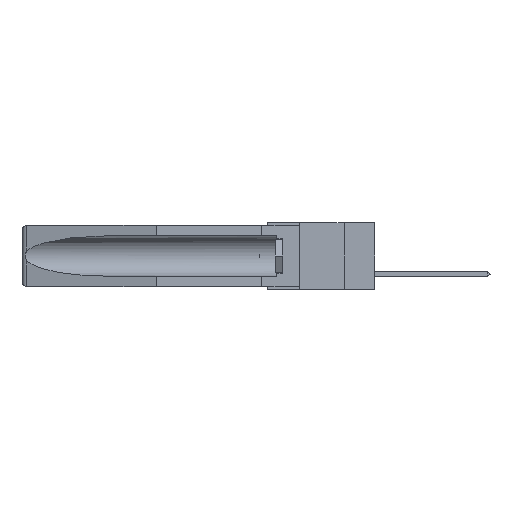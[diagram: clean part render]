
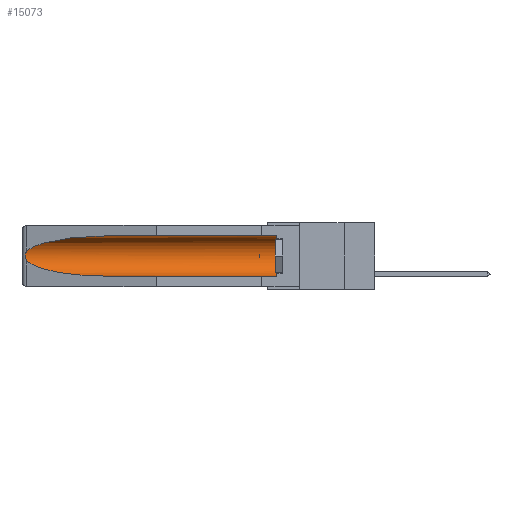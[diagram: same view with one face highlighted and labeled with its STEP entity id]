
A CAD part, left-side view. The second image highlights one B-rep face of the part: STEP entity #15073.
In plain terms, the highlighted cylindrical face has radius 2.857 mm (diameter 5.715 mm), a partial arc.
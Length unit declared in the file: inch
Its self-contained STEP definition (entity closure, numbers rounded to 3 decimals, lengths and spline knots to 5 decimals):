
#149 = CARTESIAN_POINT ( 'NONE',  ( 0.25451, 1.48313, -0.24835 ) ) ;
#455 =( BOUNDED_CURVE ( )  B_SPLINE_CURVE ( 3, ( #33222, #30406, #4039, #22581 ),
 .UNSPECIFIED., .F., .F. ) 
 B_SPLINE_CURVE_WITH_KNOTS ( ( 4, 4 ),
 ( 4.71239, 6.08839 ),
 .UNSPECIFIED. ) 
 CURVE ( )  GEOMETRIC_REPRESENTATION_ITEM ( )  RATIONAL_B_SPLINE_CURVE ( ( 1., 0.848, 0.848, 1. ) ) 
 REPRESENTATION_ITEM ( '' )  );
#1228 = VECTOR ( 'NONE', #14519, 39.37008 ) ;
#1264 = LINE ( 'NONE', #25071, #1228 ) ;
#1366 = VERTEX_POINT ( 'NONE', #9580 ) ;
#1569 = CARTESIAN_POINT ( 'NONE',  ( 0.26597, 1.5296, -0.19026 ) ) ;
#2656 = CARTESIAN_POINT ( 'NONE',  ( 0.155, 1.07973, -0.284 ) ) ;
#2924 = VERTEX_POINT ( 'NONE', #24906 ) ;
#3995 = CARTESIAN_POINT ( 'NONE',  ( 0.26655, 1.53094, -0.18657 ) ) ;
#4039 = CARTESIAN_POINT ( 'NONE',  ( 0.25451, 1.48313, -0.09465 ) ) ;
#4229 = CARTESIAN_POINT ( 'NONE',  ( 0.26537, 1.52718, -0.19328 ) ) ;
#4507 = ORIENTED_EDGE ( 'NONE', *, *, #25026, .T. ) ;
#4706 = EDGE_CURVE ( 'NONE', #17522, #2924, #455, .T. ) ;
#6212 = CARTESIAN_POINT ( 'NONE',  ( 0.26537, 1.52718, -0.14972 ) ) ;
#7579 = EDGE_CURVE ( 'NONE', #2924, #20879, #8473, .T. ) ;
#7726 = CIRCLE ( 'NONE', #8558, 0.1125 ) ;
#8138 = EDGE_CURVE ( 'NONE', #20879, #32421, #20408, .T. ) ;
#8183 = DIRECTION ( 'NONE',  ( 0., 1., 0. ) ) ;
#8473 = B_SPLINE_CURVE_WITH_KNOTS ( 'NONE', 3,
 ( #6212, #8838, #17694, #12212, #30726, #22438, #33421, #3995, #1569, #4229 ),
 .UNSPECIFIED., .F., .F.,
 ( 4, 2, 2, 2, 4 ),
 ( 0., 0.00029, 0.00058, 0.00087, 0.00117 ),
 .UNSPECIFIED. ) ;
#8558 = AXIS2_PLACEMENT_3D ( 'NONE', #24731, #11501, #24960 ) ;
#8838 = CARTESIAN_POINT ( 'NONE',  ( 0.26597, 1.52961, -0.15275 ) ) ;
#9424 = CYLINDRICAL_SURFACE ( 'NONE', #12604, 0.1125 ) ;
#9580 = CARTESIAN_POINT ( 'NONE',  ( 0.155, 0.126, -0.284 ) ) ;
#10263 = LINE ( 'NONE', #13061, #29848 ) ;
#10371 = DIRECTION ( 'NONE',  ( 0., 1., 0. ) ) ;
#10529 = CARTESIAN_POINT ( 'NONE',  ( 0.26537, 1.52718, -0.19328 ) ) ;
#10541 = CARTESIAN_POINT ( 'NONE',  ( 0.155, 0.126, -0.059 ) ) ;
#11501 = DIRECTION ( 'NONE',  ( 0., -1., 0. ) ) ;
#12096 = CARTESIAN_POINT ( 'NONE',  ( 0.155, 1.07973, -0.284 ) ) ;
#12212 = CARTESIAN_POINT ( 'NONE',  ( 0.2673, 1.5327, -0.16383 ) ) ;
#12604 = AXIS2_PLACEMENT_3D ( 'NONE', #26667, #8183, #24227 ) ;
#12997 = ORIENTED_EDGE ( 'NONE', *, *, #23770, .F. ) ;
#13061 = CARTESIAN_POINT ( 'NONE',  ( 0.155, -0.30754, -0.059 ) ) ;
#14245 = ORIENTED_EDGE ( 'NONE', *, *, #4706, .T. ) ;
#14519 = DIRECTION ( 'NONE',  ( 0., 1., 0. ) ) ;
#15073 = ADVANCED_FACE ( 'NONE', ( #21075 ), #9424, .F. ) ;
#17522 = VERTEX_POINT ( 'NONE', #18012 ) ;
#17694 = CARTESIAN_POINT ( 'NONE',  ( 0.26654, 1.53092, -0.15636 ) ) ;
#18012 = CARTESIAN_POINT ( 'NONE',  ( 0.155, 1.07973, -0.059 ) ) ;
#20408 =( BOUNDED_CURVE ( )  B_SPLINE_CURVE ( 3, ( #10529, #149, #29161, #2656 ),
 .UNSPECIFIED., .F., .F. ) 
 B_SPLINE_CURVE_WITH_KNOTS ( ( 4, 4 ),
 ( 0.1948, 1.5708 ),
 .UNSPECIFIED. ) 
 CURVE ( )  GEOMETRIC_REPRESENTATION_ITEM ( )  RATIONAL_B_SPLINE_CURVE ( ( 1., 0.848, 0.848, 1. ) ) 
 REPRESENTATION_ITEM ( '' )  );
#20879 = VERTEX_POINT ( 'NONE', #24384 ) ;
#21075 = FACE_OUTER_BOUND ( 'NONE', #24637, .T. ) ;
#22438 = CARTESIAN_POINT ( 'NONE',  ( 0.2675, 1.53308, -0.17534 ) ) ;
#22581 = CARTESIAN_POINT ( 'NONE',  ( 0.26537, 1.52718, -0.14972 ) ) ;
#23770 = EDGE_CURVE ( 'NONE', #1366, #32421, #1264, .T. ) ;
#24227 = DIRECTION ( 'NONE',  ( 0., 0., 1. ) ) ;
#24384 = CARTESIAN_POINT ( 'NONE',  ( 0.26537, 1.52718, -0.19328 ) ) ;
#24637 = EDGE_LOOP ( 'NONE', ( #14245, #26357, #29090, #12997, #4507, #30408 ) ) ;
#24731 = CARTESIAN_POINT ( 'NONE',  ( 0.155, 0.126, -0.1715 ) ) ;
#24906 = CARTESIAN_POINT ( 'NONE',  ( 0.26537, 1.52718, -0.14972 ) ) ;
#24960 = DIRECTION ( 'NONE',  ( 0., 0., 1. ) ) ;
#25026 = EDGE_CURVE ( 'NONE', #1366, #25907, #7726, .T. ) ;
#25071 = CARTESIAN_POINT ( 'NONE',  ( 0.155, -0.30754, -0.284 ) ) ;
#25907 = VERTEX_POINT ( 'NONE', #10541 ) ;
#26357 = ORIENTED_EDGE ( 'NONE', *, *, #7579, .T. ) ;
#26667 = CARTESIAN_POINT ( 'NONE',  ( 0.155, -0.30754, -0.1715 ) ) ;
#26772 = EDGE_CURVE ( 'NONE', #25907, #17522, #10263, .T. ) ;
#29090 = ORIENTED_EDGE ( 'NONE', *, *, #8138, .T. ) ;
#29161 = CARTESIAN_POINT ( 'NONE',  ( 0.21114, 1.30732, -0.284 ) ) ;
#29848 = VECTOR ( 'NONE', #10371, 39.37008 ) ;
#30406 = CARTESIAN_POINT ( 'NONE',  ( 0.21114, 1.30732, -0.059 ) ) ;
#30408 = ORIENTED_EDGE ( 'NONE', *, *, #26772, .T. ) ;
#30726 = CARTESIAN_POINT ( 'NONE',  ( 0.2675, 1.53308, -0.16763 ) ) ;
#32421 = VERTEX_POINT ( 'NONE', #12096 ) ;
#33222 = CARTESIAN_POINT ( 'NONE',  ( 0.155, 1.07973, -0.059 ) ) ;
#33421 = CARTESIAN_POINT ( 'NONE',  ( 0.2673, 1.53269, -0.17917 ) ) ;
